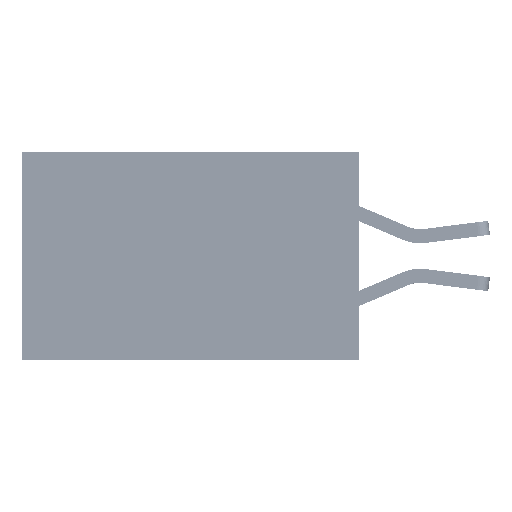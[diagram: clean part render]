
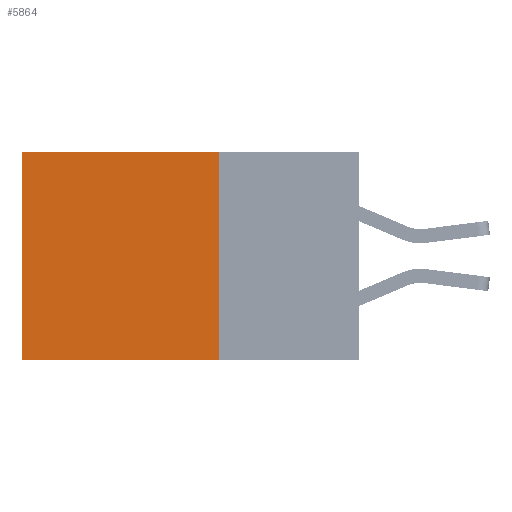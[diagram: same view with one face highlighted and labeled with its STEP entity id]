
A CAD part, left-side view. The second image highlights one B-rep face of the part: STEP entity #5864.
In plain terms, the highlighted planar face has unit normal (-1, 0, 0).
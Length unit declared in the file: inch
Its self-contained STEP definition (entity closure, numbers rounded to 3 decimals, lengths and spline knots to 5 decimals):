
#193 = VECTOR ( 'NONE', #38239, 39.37008 ) ;
#875 = CARTESIAN_POINT ( 'NONE',  ( 0.2875, 0.25, 0. ) ) ;
#1475 = LINE ( 'NONE', #875, #8753 ) ;
#3205 = CARTESIAN_POINT ( 'NONE',  ( 0.2875, 0.6, 0. ) ) ;
#3649 = ORIENTED_EDGE ( 'NONE', *, *, #15676, .F. ) ;
#4471 = CARTESIAN_POINT ( 'NONE',  ( 0.2875, 0.25, -0.37 ) ) ;
#5272 = ORIENTED_EDGE ( 'NONE', *, *, #15942, .T. ) ;
#5428 = VERTEX_POINT ( 'NONE', #8569 ) ;
#5864 = ADVANCED_FACE ( 'NONE', ( #8122 ), #20355, .F. ) ;
#7800 = LINE ( 'NONE', #10214, #193 ) ;
#8122 = FACE_OUTER_BOUND ( 'NONE', #11274, .T. ) ;
#8569 = CARTESIAN_POINT ( 'NONE',  ( 0.2875, 0.6, -0.37 ) ) ;
#8753 = VECTOR ( 'NONE', #37555, 39.37008 ) ;
#9904 = DIRECTION ( 'NONE',  ( 0., 1., 0. ) ) ;
#10201 = EDGE_CURVE ( 'NONE', #17878, #5428, #34334, .T. ) ;
#10214 = CARTESIAN_POINT ( 'NONE',  ( 0.2875, 0.25, 0. ) ) ;
#11274 = EDGE_LOOP ( 'NONE', ( #5272, #19285, #3649, #28572 ) ) ;
#11321 = DIRECTION ( 'NONE',  ( 0., 0., -1. ) ) ;
#14543 = CARTESIAN_POINT ( 'NONE',  ( 0.2875, 0.25, 0. ) ) ;
#14766 = VERTEX_POINT ( 'NONE', #28682 ) ;
#15676 = EDGE_CURVE ( 'NONE', #14766, #17878, #1475, .T. ) ;
#15942 = EDGE_CURVE ( 'NONE', #16475, #5428, #33914, .T. ) ;
#16475 = VERTEX_POINT ( 'NONE', #3205 ) ;
#17878 = VERTEX_POINT ( 'NONE', #28263 ) ;
#18963 = EDGE_CURVE ( 'NONE', #14766, #16475, #7800, .T. ) ;
#19285 = ORIENTED_EDGE ( 'NONE', *, *, #10201, .F. ) ;
#20355 = PLANE ( 'NONE',  #26949 ) ;
#24508 = DIRECTION ( 'NONE',  ( 0., 0., -1. ) ) ;
#26557 = DIRECTION ( 'NONE',  ( 1., 0., 0. ) ) ;
#26949 = AXIS2_PLACEMENT_3D ( 'NONE', #14543, #26557, #11321 ) ;
#27312 = CARTESIAN_POINT ( 'NONE',  ( 0.2875, 0.6, 0. ) ) ;
#28263 = CARTESIAN_POINT ( 'NONE',  ( 0.2875, 0.25, -0.37 ) ) ;
#28572 = ORIENTED_EDGE ( 'NONE', *, *, #18963, .T. ) ;
#28682 = CARTESIAN_POINT ( 'NONE',  ( 0.2875, 0.25, 0. ) ) ;
#33214 = VECTOR ( 'NONE', #9904, 39.37008 ) ;
#33914 = LINE ( 'NONE', #27312, #38966 ) ;
#34334 = LINE ( 'NONE', #4471, #33214 ) ;
#37555 = DIRECTION ( 'NONE',  ( 0., 0., -1. ) ) ;
#38239 = DIRECTION ( 'NONE',  ( 0., 1., 0. ) ) ;
#38966 = VECTOR ( 'NONE', #24508, 39.37008 ) ;
